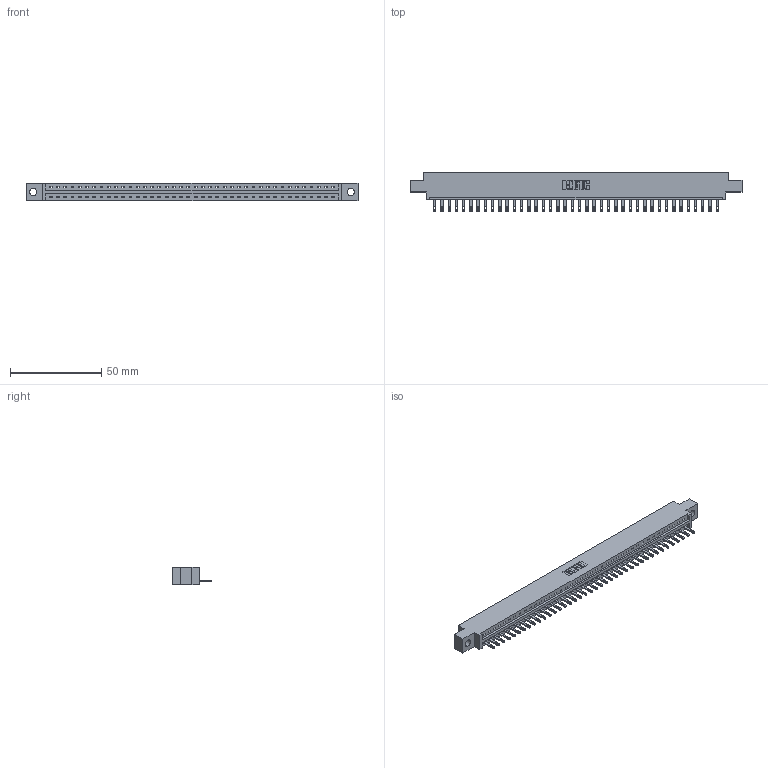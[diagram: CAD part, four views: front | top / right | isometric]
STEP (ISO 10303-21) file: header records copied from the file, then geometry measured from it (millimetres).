
FILE_DESCRIPTION (( 'STEP AP203' ), '1' );
FILE_NAME ('887-040-500-604.STEP', '2020-09-20T23:28:20', ( '' ), ( '' ), 'SwSTEP 2.0', 'SolidWorks 2020', '' );
FILE_SCHEMA (( 'CONFIG_CONTROL_DESIGN' ));
Length unit declared in the file: inch
Products named in the file (3): 345-292-001_345-293-100; 887-040-500-604; 837 Part_0.170 Offset - 0.156 Dia-TH
Assembly tree (41 placements, depth 2):
  887-040-500-604
    837 Part_0.170 Offset - 0.156 Dia-TH
    345-292-001_345-293-100  x40
Bounding box: 181.51 x 21.85 x 9.4 mm (x, y, z)
Volume: 18659.1 mm3; surface area: 19255.4 mm2
Topology: 41 solids, 41 shells, 2438 faces, 7523 edges, 5014 vertices
Faces by surface type: plane 1674, cylinder 764
Entity records: 30057 total; most frequent: CARTESIAN_POINT 5242, ORIENTED_EDGE 5218, DIRECTION 4417, EDGE_CURVE 2609, VECTOR 2477, LINE 2477, VERTEX_POINT 1738, AXIS2_PLACEMENT_3D 970
